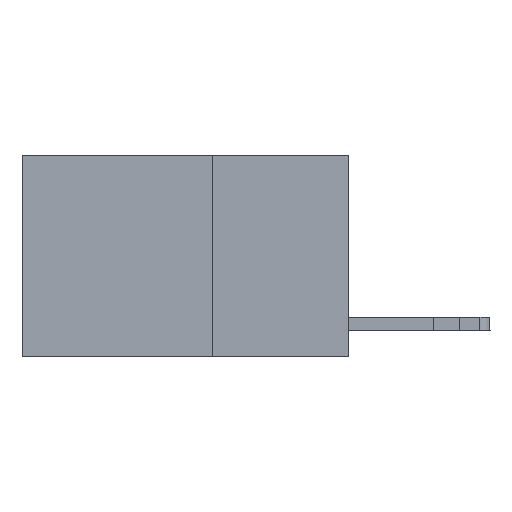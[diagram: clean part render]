
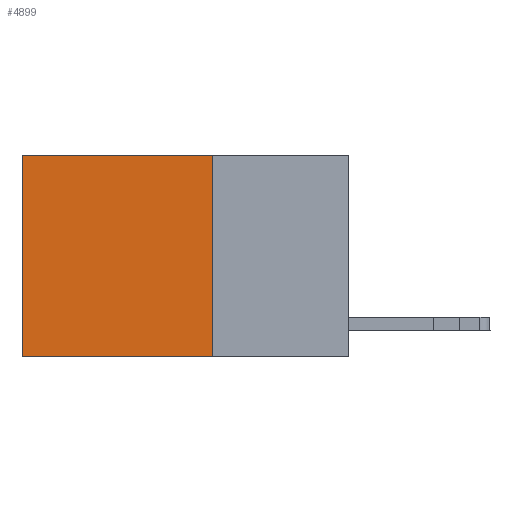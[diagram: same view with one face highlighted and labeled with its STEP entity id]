
A CAD part, left-side view. The second image highlights one B-rep face of the part: STEP entity #4899.
In plain terms, the highlighted planar face has unit normal (-1, 0, 0).
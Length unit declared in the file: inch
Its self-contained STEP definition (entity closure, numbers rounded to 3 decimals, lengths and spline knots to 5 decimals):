
#911 = CARTESIAN_POINT ( 'NONE',  ( 0.2625, 0.6, 0. ) ) ;
#1148 = DIRECTION ( 'NONE',  ( 0., 0., -1. ) ) ;
#1166 = PLANE ( 'NONE',  #14148 ) ;
#1206 = ORIENTED_EDGE ( 'NONE', *, *, #5515, .F. ) ;
#1674 = CARTESIAN_POINT ( 'NONE',  ( 0.2625, 0.25, -0.37 ) ) ;
#3651 = CARTESIAN_POINT ( 'NONE',  ( 0.2625, 0.6, 0. ) ) ;
#4073 = CARTESIAN_POINT ( 'NONE',  ( 0.2625, 0.25, 0. ) ) ;
#4239 = LINE ( 'NONE', #4073, #9747 ) ;
#4899 = ADVANCED_FACE ( 'NONE', ( #13673 ), #1166, .F. ) ;
#4967 = ORIENTED_EDGE ( 'NONE', *, *, #9435, .F. ) ;
#5002 = VECTOR ( 'NONE', #1148, 39.37008 ) ;
#5443 = LINE ( 'NONE', #9284, #16221 ) ;
#5515 = EDGE_CURVE ( 'NONE', #9533, #12162, #5443, .T. ) ;
#6912 = CARTESIAN_POINT ( 'NONE',  ( 0.2625, 0.25, -0.37 ) ) ;
#7816 = EDGE_CURVE ( 'NONE', #15406, #10409, #8556, .T. ) ;
#8155 = VECTOR ( 'NONE', #16240, 39.37008 ) ;
#8556 = LINE ( 'NONE', #911, #5002 ) ;
#9284 = CARTESIAN_POINT ( 'NONE',  ( 0.2625, 0.25, 0. ) ) ;
#9392 = EDGE_CURVE ( 'NONE', #9533, #15406, #4239, .T. ) ;
#9435 = EDGE_CURVE ( 'NONE', #12162, #10409, #12956, .T. ) ;
#9533 = VERTEX_POINT ( 'NONE', #15226 ) ;
#9620 = ORIENTED_EDGE ( 'NONE', *, *, #9392, .T. ) ;
#9643 = DIRECTION ( 'NONE',  ( 0., 0., -1. ) ) ;
#9747 = VECTOR ( 'NONE', #14268, 39.37008 ) ;
#9898 = ORIENTED_EDGE ( 'NONE', *, *, #7816, .T. ) ;
#10409 = VERTEX_POINT ( 'NONE', #12959 ) ;
#10528 = DIRECTION ( 'NONE',  ( 0., 0., -1. ) ) ;
#10877 = CARTESIAN_POINT ( 'NONE',  ( 0.2625, 0.25, 0. ) ) ;
#11883 = EDGE_LOOP ( 'NONE', ( #9898, #4967, #1206, #9620 ) ) ;
#12162 = VERTEX_POINT ( 'NONE', #6912 ) ;
#12956 = LINE ( 'NONE', #1674, #8155 ) ;
#12959 = CARTESIAN_POINT ( 'NONE',  ( 0.2625, 0.6, -0.37 ) ) ;
#13673 = FACE_OUTER_BOUND ( 'NONE', #11883, .T. ) ;
#14148 = AXIS2_PLACEMENT_3D ( 'NONE', #10877, #15930, #9643 ) ;
#14268 = DIRECTION ( 'NONE',  ( 0., 1., 0. ) ) ;
#15226 = CARTESIAN_POINT ( 'NONE',  ( 0.2625, 0.25, 0. ) ) ;
#15406 = VERTEX_POINT ( 'NONE', #3651 ) ;
#15930 = DIRECTION ( 'NONE',  ( 1., 0., 0. ) ) ;
#16221 = VECTOR ( 'NONE', #10528, 39.37008 ) ;
#16240 = DIRECTION ( 'NONE',  ( 0., 1., 0. ) ) ;
